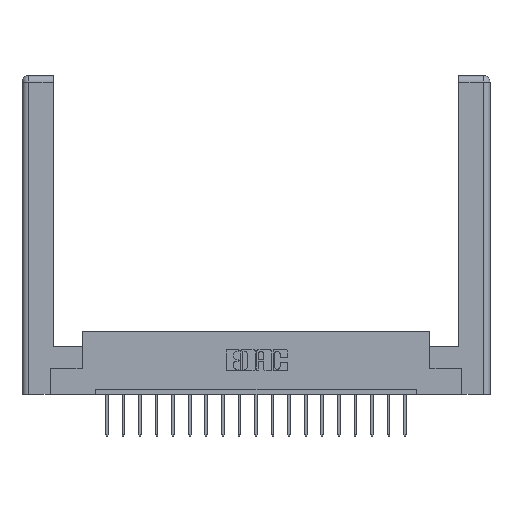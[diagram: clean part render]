
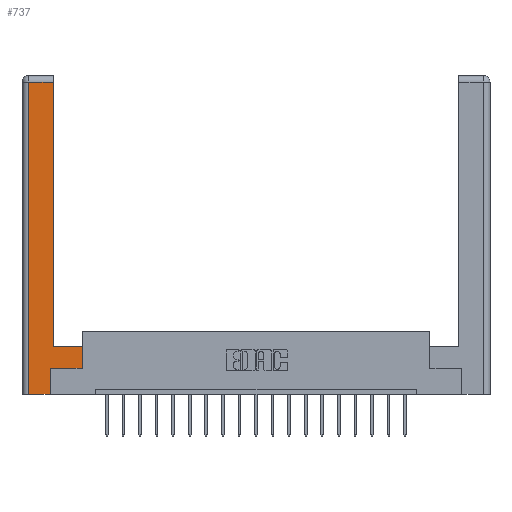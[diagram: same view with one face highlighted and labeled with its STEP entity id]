
A CAD part, top view. The second image highlights one B-rep face of the part: STEP entity #737.
In plain terms, the highlighted planar face has unit normal (0, 0, 1).
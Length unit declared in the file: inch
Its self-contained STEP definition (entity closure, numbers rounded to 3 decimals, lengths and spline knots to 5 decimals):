
#528 = CARTESIAN_POINT ( 'NONE',  ( 0.295, 0.45, 0. ) ) ;
#737 = ADVANCED_FACE ( 'NONE', ( #9213 ), #18674, .F. ) ;
#851 = DIRECTION ( 'NONE',  ( 1., 0., 0. ) ) ;
#854 = EDGE_LOOP ( 'NONE', ( #5282, #18196, #6168, #2160, #14659, #14344, #4450, #13929 ) ) ;
#1218 = VECTOR ( 'NONE', #851, 39.37008 ) ;
#2160 = ORIENTED_EDGE ( 'NONE', *, *, #8052, .T. ) ;
#3450 = LINE ( 'NONE', #7189, #12751 ) ;
#4027 = CARTESIAN_POINT ( 'NONE',  ( 0.565, 0.45, 0. ) ) ;
#4067 = DIRECTION ( 'NONE',  ( 1., 0., 0. ) ) ;
#4116 = LINE ( 'NONE', #9032, #5059 ) ;
#4312 = VECTOR ( 'NONE', #15597, 39.37008 ) ;
#4450 = ORIENTED_EDGE ( 'NONE', *, *, #7633, .T. ) ;
#4714 = CARTESIAN_POINT ( 'NONE',  ( 0.295, 2.94, 0. ) ) ;
#4788 = EDGE_CURVE ( 'NONE', #16647, #6243, #8072, .T. ) ;
#4909 = VERTEX_POINT ( 'NONE', #11580 ) ;
#5059 = VECTOR ( 'NONE', #15007, 39.37008 ) ;
#5093 = VECTOR ( 'NONE', #18928, 39.37008 ) ;
#5282 = ORIENTED_EDGE ( 'NONE', *, *, #9776, .T. ) ;
#5729 = DIRECTION ( 'NONE',  ( -1., 0., 0. ) ) ;
#5825 = CARTESIAN_POINT ( 'NONE',  ( 0.0615, 0., 0. ) ) ;
#5894 = CARTESIAN_POINT ( 'NONE',  ( 0.265, 0.245, 0. ) ) ;
#6168 = ORIENTED_EDGE ( 'NONE', *, *, #6666, .T. ) ;
#6243 = VERTEX_POINT ( 'NONE', #8557 ) ;
#6348 = DIRECTION ( 'NONE',  ( 0., 1., 0. ) ) ;
#6513 = VERTEX_POINT ( 'NONE', #4027 ) ;
#6538 = VERTEX_POINT ( 'NONE', #14695 ) ;
#6666 = EDGE_CURVE ( 'NONE', #19240, #4909, #12311, .T. ) ;
#7189 = CARTESIAN_POINT ( 'NONE',  ( 0.0615, 2.94, 0. ) ) ;
#7633 = EDGE_CURVE ( 'NONE', #15285, #6513, #17789, .T. ) ;
#7991 = EDGE_CURVE ( 'NONE', #13752, #19240, #3450, .T. ) ;
#8052 = EDGE_CURVE ( 'NONE', #4909, #16647, #14204, .T. ) ;
#8072 = LINE ( 'NONE', #5894, #4312 ) ;
#8557 = CARTESIAN_POINT ( 'NONE',  ( 0.265, 0.245, 0. ) ) ;
#8664 = DIRECTION ( 'NONE',  ( 0., -1., 0. ) ) ;
#9015 = EDGE_CURVE ( 'NONE', #6513, #6538, #9607, .T. ) ;
#9032 = CARTESIAN_POINT ( 'NONE',  ( 0.295, 3., 0. ) ) ;
#9213 = FACE_OUTER_BOUND ( 'NONE', #854, .T. ) ;
#9538 = DIRECTION ( 'NONE',  ( 0., 0., -1. ) ) ;
#9607 = LINE ( 'NONE', #528, #5093 ) ;
#9676 = VECTOR ( 'NONE', #8664, 39.37008 ) ;
#9776 = EDGE_CURVE ( 'NONE', #6538, #13752, #4116, .T. ) ;
#10384 = VECTOR ( 'NONE', #4067, 39.37008 ) ;
#10508 = LINE ( 'NONE', #19033, #1218 ) ;
#11580 = CARTESIAN_POINT ( 'NONE',  ( 0.0615, 0., 0. ) ) ;
#12236 = EDGE_CURVE ( 'NONE', #6243, #15285, #10508, .T. ) ;
#12290 = VECTOR ( 'NONE', #6348, 39.37008 ) ;
#12311 = LINE ( 'NONE', #5825, #9676 ) ;
#12743 = CARTESIAN_POINT ( 'NONE',  ( 0., 0., 0. ) ) ;
#12751 = VECTOR ( 'NONE', #5729, 39.37008 ) ;
#13208 = CARTESIAN_POINT ( 'NONE',  ( 0.265, 0., 0. ) ) ;
#13752 = VERTEX_POINT ( 'NONE', #4714 ) ;
#13929 = ORIENTED_EDGE ( 'NONE', *, *, #9015, .T. ) ;
#14004 = AXIS2_PLACEMENT_3D ( 'NONE', #12743, #9538, #15901 ) ;
#14204 = LINE ( 'NONE', #13208, #10384 ) ;
#14344 = ORIENTED_EDGE ( 'NONE', *, *, #12236, .T. ) ;
#14659 = ORIENTED_EDGE ( 'NONE', *, *, #4788, .T. ) ;
#14695 = CARTESIAN_POINT ( 'NONE',  ( 0.295, 0.45, 0. ) ) ;
#14726 = CARTESIAN_POINT ( 'NONE',  ( 0.0615, 2.94, 0. ) ) ;
#15007 = DIRECTION ( 'NONE',  ( 0., 1., 0. ) ) ;
#15118 = CARTESIAN_POINT ( 'NONE',  ( 0.265, 0., 0. ) ) ;
#15285 = VERTEX_POINT ( 'NONE', #16645 ) ;
#15597 = DIRECTION ( 'NONE',  ( 0., 1., 0. ) ) ;
#15901 = DIRECTION ( 'NONE',  ( -1., 0., 0. ) ) ;
#16645 = CARTESIAN_POINT ( 'NONE',  ( 0.565, 0.245, 0. ) ) ;
#16647 = VERTEX_POINT ( 'NONE', #15118 ) ;
#17789 = LINE ( 'NONE', #18344, #12290 ) ;
#18196 = ORIENTED_EDGE ( 'NONE', *, *, #7991, .T. ) ;
#18344 = CARTESIAN_POINT ( 'NONE',  ( 0.565, 0.45, 0. ) ) ;
#18674 = PLANE ( 'NONE',  #14004 ) ;
#18928 = DIRECTION ( 'NONE',  ( -1., 0., 0. ) ) ;
#19033 = CARTESIAN_POINT ( 'NONE',  ( 0.565, 0.245, 0. ) ) ;
#19240 = VERTEX_POINT ( 'NONE', #14726 ) ;
